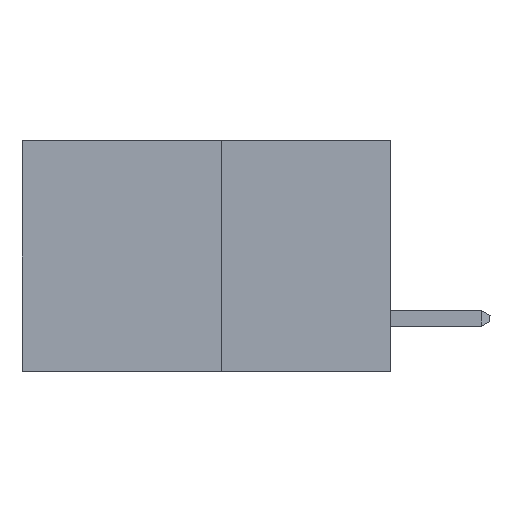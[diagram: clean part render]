
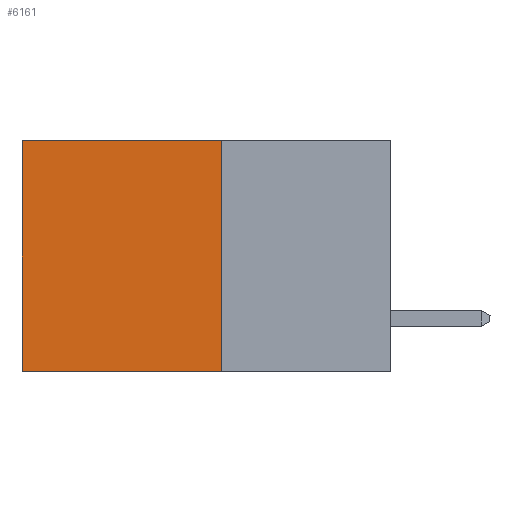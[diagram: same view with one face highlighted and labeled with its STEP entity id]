
A CAD part, left-side view. The second image highlights one B-rep face of the part: STEP entity #6161.
In plain terms, the highlighted planar face has unit normal (-1, 0, 0).
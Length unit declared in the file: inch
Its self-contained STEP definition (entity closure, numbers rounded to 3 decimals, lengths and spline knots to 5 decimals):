
#539 = ORIENTED_EDGE ( 'NONE', *, *, #3772, .T. ) ;
#654 = LINE ( 'NONE', #6863, #7724 ) ;
#878 = CARTESIAN_POINT ( 'NONE',  ( 0.277, 0.59, -0.37 ) ) ;
#1142 = CARTESIAN_POINT ( 'NONE',  ( 0.277, 0.59, 0. ) ) ;
#1923 = CARTESIAN_POINT ( 'NONE',  ( 0.277, 0.27, -0.37 ) ) ;
#2257 = EDGE_CURVE ( 'NONE', #10933, #6147, #2746, .T. ) ;
#2266 = VERTEX_POINT ( 'NONE', #10055 ) ;
#2444 = EDGE_CURVE ( 'NONE', #2266, #2626, #654, .T. ) ;
#2465 = EDGE_LOOP ( 'NONE', ( #7417, #5803, #2562, #539 ) ) ;
#2562 = ORIENTED_EDGE ( 'NONE', *, *, #2444, .F. ) ;
#2626 = VERTEX_POINT ( 'NONE', #3216 ) ;
#2746 = LINE ( 'NONE', #10127, #7225 ) ;
#2902 = DIRECTION ( 'NONE',  ( 1., 0., 0. ) ) ;
#3216 = CARTESIAN_POINT ( 'NONE',  ( 0.277, 0.27, -0.37 ) ) ;
#3772 = EDGE_CURVE ( 'NONE', #2266, #10933, #5456, .T. ) ;
#4371 = EDGE_CURVE ( 'NONE', #2626, #6147, #7176, .T. ) ;
#5456 = LINE ( 'NONE', #11280, #9805 ) ;
#5803 = ORIENTED_EDGE ( 'NONE', *, *, #4371, .F. ) ;
#6147 = VERTEX_POINT ( 'NONE', #878 ) ;
#6161 = ADVANCED_FACE ( 'NONE', ( #6333 ), #8154, .F. ) ;
#6333 = FACE_OUTER_BOUND ( 'NONE', #2465, .T. ) ;
#6520 = DIRECTION ( 'NONE',  ( 0., 1., 0. ) ) ;
#6751 = DIRECTION ( 'NONE',  ( 0., 0., -1. ) ) ;
#6863 = CARTESIAN_POINT ( 'NONE',  ( 0.277, 0.27, -0.37 ) ) ;
#6910 = VECTOR ( 'NONE', #8750, 39.37008 ) ;
#7176 = LINE ( 'NONE', #7958, #6910 ) ;
#7225 = VECTOR ( 'NONE', #10078, 39.37008 ) ;
#7417 = ORIENTED_EDGE ( 'NONE', *, *, #2257, .T. ) ;
#7724 = VECTOR ( 'NONE', #6751, 39.37008 ) ;
#7958 = CARTESIAN_POINT ( 'NONE',  ( 0.277, 0.27, -0.37 ) ) ;
#8154 = PLANE ( 'NONE',  #9841 ) ;
#8750 = DIRECTION ( 'NONE',  ( 0., 1., 0. ) ) ;
#8957 = DIRECTION ( 'NONE',  ( 0., 0., -1. ) ) ;
#9805 = VECTOR ( 'NONE', #6520, 39.37008 ) ;
#9841 = AXIS2_PLACEMENT_3D ( 'NONE', #1923, #2902, #8957 ) ;
#10055 = CARTESIAN_POINT ( 'NONE',  ( 0.277, 0.27, 0. ) ) ;
#10078 = DIRECTION ( 'NONE',  ( 0., 0., -1. ) ) ;
#10127 = CARTESIAN_POINT ( 'NONE',  ( 0.277, 0.59, -0.37 ) ) ;
#10933 = VERTEX_POINT ( 'NONE', #1142 ) ;
#11280 = CARTESIAN_POINT ( 'NONE',  ( 0.277, 0.27, 0. ) ) ;
